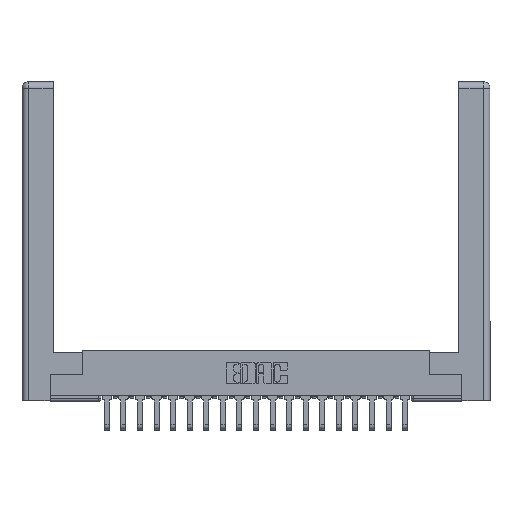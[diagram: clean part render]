
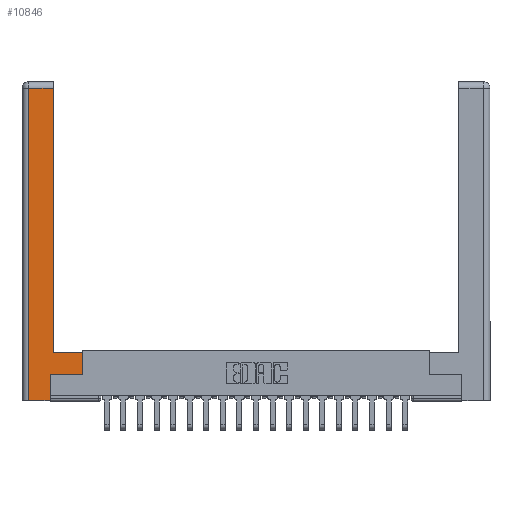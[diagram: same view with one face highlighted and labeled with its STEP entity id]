
A CAD part, top view. The second image highlights one B-rep face of the part: STEP entity #10846.
In plain terms, the highlighted planar face has unit normal (0, 0, 1).
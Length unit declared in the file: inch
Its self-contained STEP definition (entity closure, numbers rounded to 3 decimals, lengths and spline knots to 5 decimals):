
#71 = VECTOR ( 'NONE', #14103, 39.37008 ) ;
#800 = CARTESIAN_POINT ( 'NONE',  ( 0.565, 0.45, 0. ) ) ;
#846 = ORIENTED_EDGE ( 'NONE', *, *, #19850, .T. ) ;
#892 = DIRECTION ( 'NONE',  ( 0., 1., 0. ) ) ;
#1583 = EDGE_CURVE ( 'NONE', #13962, #9497, #11405, .T. ) ;
#1753 = LINE ( 'NONE', #5078, #14730 ) ;
#2789 = VECTOR ( 'NONE', #12789, 39.37008 ) ;
#2853 = ORIENTED_EDGE ( 'NONE', *, *, #3652, .T. ) ;
#3553 = ORIENTED_EDGE ( 'NONE', *, *, #3869, .T. ) ;
#3566 = LINE ( 'NONE', #11064, #2789 ) ;
#3652 = EDGE_CURVE ( 'NONE', #18482, #8017, #13598, .T. ) ;
#3842 = DIRECTION ( 'NONE',  ( -1., 0., 0. ) ) ;
#3869 = EDGE_CURVE ( 'NONE', #13217, #13962, #18602, .T. ) ;
#4393 = EDGE_CURVE ( 'NONE', #9497, #18482, #12744, .T. ) ;
#4681 = ORIENTED_EDGE ( 'NONE', *, *, #4393, .T. ) ;
#4689 = CARTESIAN_POINT ( 'NONE',  ( 0.265, 0.245, 0. ) ) ;
#4786 = CARTESIAN_POINT ( 'NONE',  ( 0.565, 0.245, 0. ) ) ;
#5078 = CARTESIAN_POINT ( 'NONE',  ( 0.265, 0., 0. ) ) ;
#5324 = DIRECTION ( 'NONE',  ( -1., 0., 0. ) ) ;
#5329 = CARTESIAN_POINT ( 'NONE',  ( 0.565, 0.245, 0. ) ) ;
#5748 = DIRECTION ( 'NONE',  ( -1., 0., 0. ) ) ;
#5824 = PLANE ( 'NONE',  #18151 ) ;
#6774 = CARTESIAN_POINT ( 'NONE',  ( 0.0615, 0., 0. ) ) ;
#6878 = CARTESIAN_POINT ( 'NONE',  ( 0.295, 0.45, 0. ) ) ;
#6906 = VECTOR ( 'NONE', #14796, 39.37008 ) ;
#7263 = EDGE_CURVE ( 'NONE', #18876, #21697, #13415, .T. ) ;
#7505 = DIRECTION ( 'NONE',  ( 0., 1., 0. ) ) ;
#7577 = FACE_OUTER_BOUND ( 'NONE', #15575, .T. ) ;
#8017 = VERTEX_POINT ( 'NONE', #15168 ) ;
#8277 = CARTESIAN_POINT ( 'NONE',  ( 0.295, 2.94, 0. ) ) ;
#8559 = VECTOR ( 'NONE', #5324, 39.37008 ) ;
#9497 = VERTEX_POINT ( 'NONE', #5329 ) ;
#10037 = CARTESIAN_POINT ( 'NONE',  ( 0.0615, 2.94, 0. ) ) ;
#10085 = VECTOR ( 'NONE', #7505, 39.37008 ) ;
#10825 = CARTESIAN_POINT ( 'NONE',  ( 0.295, 3., 0. ) ) ;
#10846 = ADVANCED_FACE ( 'NONE', ( #7577 ), #5824, .F. ) ;
#11064 = CARTESIAN_POINT ( 'NONE',  ( 0.0615, 0., 0. ) ) ;
#11233 = EDGE_CURVE ( 'NONE', #20120, #13217, #1753, .T. ) ;
#11405 = LINE ( 'NONE', #4786, #6906 ) ;
#12411 = CARTESIAN_POINT ( 'NONE',  ( 0.265, 0., 0. ) ) ;
#12744 = LINE ( 'NONE', #800, #10085 ) ;
#12789 = DIRECTION ( 'NONE',  ( 0., -1., 0. ) ) ;
#13217 = VERTEX_POINT ( 'NONE', #12411 ) ;
#13415 = LINE ( 'NONE', #17285, #17360 ) ;
#13598 = LINE ( 'NONE', #6878, #8559 ) ;
#13637 = ORIENTED_EDGE ( 'NONE', *, *, #15644, .T. ) ;
#13962 = VERTEX_POINT ( 'NONE', #4689 ) ;
#14103 = DIRECTION ( 'NONE',  ( 0., 1., 0. ) ) ;
#14113 = VECTOR ( 'NONE', #892, 39.37008 ) ;
#14730 = VECTOR ( 'NONE', #20308, 39.37008 ) ;
#14796 = DIRECTION ( 'NONE',  ( 1., 0., 0. ) ) ;
#15168 = CARTESIAN_POINT ( 'NONE',  ( 0.295, 0.45, 0. ) ) ;
#15575 = EDGE_LOOP ( 'NONE', ( #13637, #20242, #846, #16409, #3553, #18843, #4681, #2853 ) ) ;
#15644 = EDGE_CURVE ( 'NONE', #8017, #18876, #19350, .T. ) ;
#16409 = ORIENTED_EDGE ( 'NONE', *, *, #11233, .T. ) ;
#17285 = CARTESIAN_POINT ( 'NONE',  ( 0.0615, 2.94, 0. ) ) ;
#17360 = VECTOR ( 'NONE', #3842, 39.37008 ) ;
#17669 = CARTESIAN_POINT ( 'NONE',  ( 0., 0., 0. ) ) ;
#18151 = AXIS2_PLACEMENT_3D ( 'NONE', #17669, #20902, #5748 ) ;
#18482 = VERTEX_POINT ( 'NONE', #20299 ) ;
#18602 = LINE ( 'NONE', #21129, #14113 ) ;
#18843 = ORIENTED_EDGE ( 'NONE', *, *, #1583, .T. ) ;
#18876 = VERTEX_POINT ( 'NONE', #8277 ) ;
#19350 = LINE ( 'NONE', #10825, #71 ) ;
#19850 = EDGE_CURVE ( 'NONE', #21697, #20120, #3566, .T. ) ;
#20120 = VERTEX_POINT ( 'NONE', #6774 ) ;
#20242 = ORIENTED_EDGE ( 'NONE', *, *, #7263, .T. ) ;
#20299 = CARTESIAN_POINT ( 'NONE',  ( 0.565, 0.45, 0. ) ) ;
#20308 = DIRECTION ( 'NONE',  ( 1., 0., 0. ) ) ;
#20902 = DIRECTION ( 'NONE',  ( 0., 0., -1. ) ) ;
#21129 = CARTESIAN_POINT ( 'NONE',  ( 0.265, 0.245, 0. ) ) ;
#21697 = VERTEX_POINT ( 'NONE', #10037 ) ;
